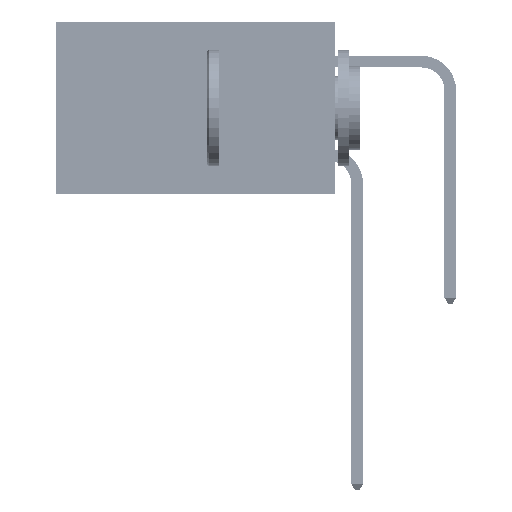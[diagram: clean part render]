
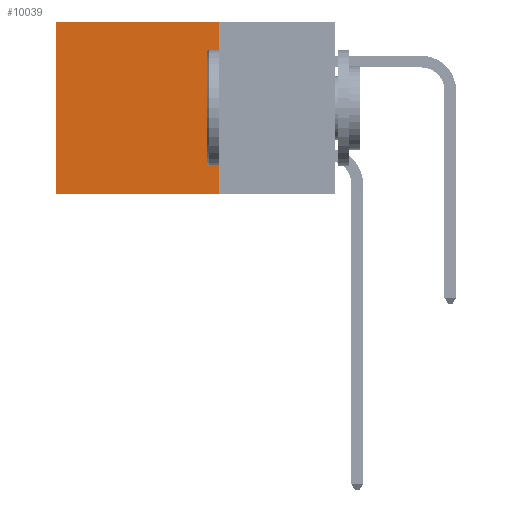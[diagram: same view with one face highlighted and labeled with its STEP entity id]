
A CAD part, left-side view. The second image highlights one B-rep face of the part: STEP entity #10039.
In plain terms, the highlighted planar face has unit normal (-1, 0, 0).
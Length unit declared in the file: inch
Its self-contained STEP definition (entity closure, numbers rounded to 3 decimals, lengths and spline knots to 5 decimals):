
#1823 = AXIS2_PLACEMENT_3D ( 'NONE', #39716, #7148, #10802 ) ;
#2929 = VERTEX_POINT ( 'NONE', #20034 ) ;
#4016 = ORIENTED_EDGE ( 'NONE', *, *, #15516, .T. ) ;
#4888 = DIRECTION ( 'NONE',  ( 0., 0., -1. ) ) ;
#7027 = DIRECTION ( 'NONE',  ( 0., 1., 0. ) ) ;
#7148 = DIRECTION ( 'NONE',  ( 1., 0., 0. ) ) ;
#8137 = VERTEX_POINT ( 'NONE', #30380 ) ;
#8266 = LINE ( 'NONE', #22401, #39987 ) ;
#10039 = ADVANCED_FACE ( 'NONE', ( #32464 ), #14616, .F. ) ;
#10802 = DIRECTION ( 'NONE',  ( 0., 0., -1. ) ) ;
#11601 = EDGE_CURVE ( 'NONE', #8137, #2929, #14901, .T. ) ;
#14616 = PLANE ( 'NONE',  #1823 ) ;
#14901 = LINE ( 'NONE', #24242, #20733 ) ;
#15516 = EDGE_CURVE ( 'NONE', #35392, #35271, #34507, .T. ) ;
#15933 = ORIENTED_EDGE ( 'NONE', *, *, #42257, .F. ) ;
#17834 = CARTESIAN_POINT ( 'NONE',  ( 0.2875, 0.6, 0. ) ) ;
#18205 = ORIENTED_EDGE ( 'NONE', *, *, #11601, .F. ) ;
#19955 = EDGE_CURVE ( 'NONE', #35271, #2929, #8266, .T. ) ;
#20034 = CARTESIAN_POINT ( 'NONE',  ( 0.2875, 0.6, -0.37 ) ) ;
#20733 = VECTOR ( 'NONE', #23686, 39.37008 ) ;
#22401 = CARTESIAN_POINT ( 'NONE',  ( 0.2875, 0.6, 0. ) ) ;
#23686 = DIRECTION ( 'NONE',  ( 0., 1., 0. ) ) ;
#24242 = CARTESIAN_POINT ( 'NONE',  ( 0.2875, 0.25, -0.37 ) ) ;
#28128 = VECTOR ( 'NONE', #7027, 39.37008 ) ;
#30380 = CARTESIAN_POINT ( 'NONE',  ( 0.2875, 0.25, -0.37 ) ) ;
#30504 = DIRECTION ( 'NONE',  ( 0., 0., -1. ) ) ;
#31782 = CARTESIAN_POINT ( 'NONE',  ( 0.2875, 0.25, 0. ) ) ;
#32464 = FACE_OUTER_BOUND ( 'NONE', #49485, .T. ) ;
#34507 = LINE ( 'NONE', #31782, #28128 ) ;
#35271 = VERTEX_POINT ( 'NONE', #17834 ) ;
#35392 = VERTEX_POINT ( 'NONE', #51559 ) ;
#39017 = VECTOR ( 'NONE', #4888, 39.37008 ) ;
#39716 = CARTESIAN_POINT ( 'NONE',  ( 0.2875, 0.25, 0. ) ) ;
#39987 = VECTOR ( 'NONE', #30504, 39.37008 ) ;
#41810 = ORIENTED_EDGE ( 'NONE', *, *, #19955, .T. ) ;
#42257 = EDGE_CURVE ( 'NONE', #35392, #8137, #46784, .T. ) ;
#45911 = CARTESIAN_POINT ( 'NONE',  ( 0.2875, 0.25, 0. ) ) ;
#46784 = LINE ( 'NONE', #45911, #39017 ) ;
#49485 = EDGE_LOOP ( 'NONE', ( #41810, #18205, #15933, #4016 ) ) ;
#51559 = CARTESIAN_POINT ( 'NONE',  ( 0.2875, 0.25, 0. ) ) ;
